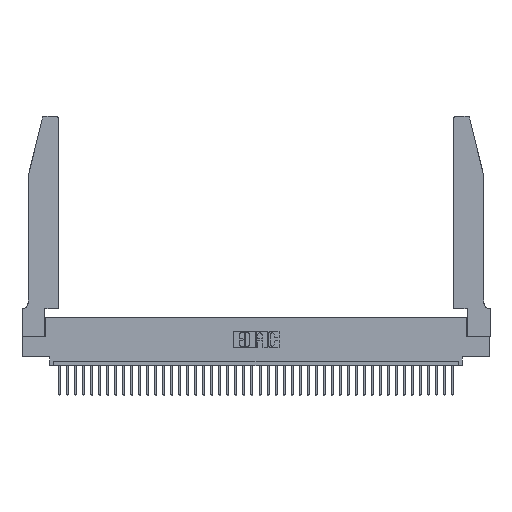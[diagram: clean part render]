
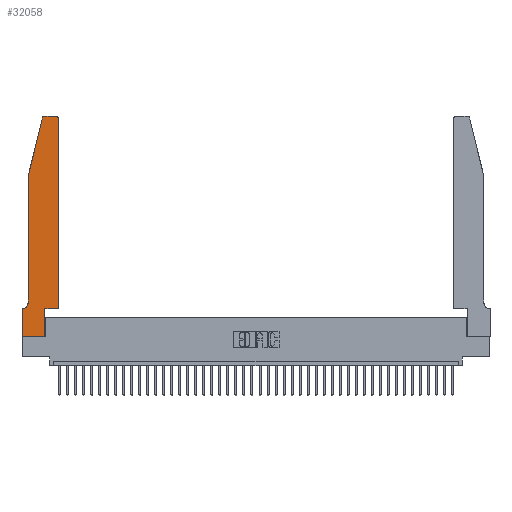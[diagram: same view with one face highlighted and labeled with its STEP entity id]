
A CAD part, top view. The second image highlights one B-rep face of the part: STEP entity #32058.
In plain terms, the highlighted planar face has unit normal (0, 0, 1).
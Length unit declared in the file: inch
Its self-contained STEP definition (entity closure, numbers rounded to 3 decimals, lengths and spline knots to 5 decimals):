
#206 = EDGE_CURVE ( 'NONE', #25502, #33551, #23242, .T. ) ;
#455 = VERTEX_POINT ( 'NONE', #18061 ) ;
#619 = VECTOR ( 'NONE', #20736, 39.37008 ) ;
#912 = EDGE_CURVE ( 'NONE', #34437, #13391, #27772, .T. ) ;
#1024 = ORIENTED_EDGE ( 'NONE', *, *, #29469, .T. ) ;
#1064 = VECTOR ( 'NONE', #20770, 39.37008 ) ;
#1552 = CARTESIAN_POINT ( 'NONE',  ( 0.2605, 2.75, 0.37 ) ) ;
#1917 = VECTOR ( 'NONE', #2538, 39.37008 ) ;
#2538 = DIRECTION ( 'NONE',  ( 0., -1., 0. ) ) ;
#2721 = VERTEX_POINT ( 'NONE', #35830 ) ;
#3305 = DIRECTION ( 'NONE',  ( 0., 0., 1. ) ) ;
#3306 = ORIENTED_EDGE ( 'NONE', *, *, #912, .T. ) ;
#3746 = CARTESIAN_POINT ( 'NONE',  ( 0., 0.35, 0.37 ) ) ;
#4103 = EDGE_CURVE ( 'NONE', #31707, #2721, #30834, .T. ) ;
#4588 = ORIENTED_EDGE ( 'NONE', *, *, #35322, .T. ) ;
#5431 = EDGE_CURVE ( 'NONE', #2721, #13974, #35699, .T. ) ;
#6191 = EDGE_CURVE ( 'NONE', #33551, #34437, #24695, .T. ) ;
#6424 = LINE ( 'NONE', #40690, #1917 ) ;
#6462 = CARTESIAN_POINT ( 'NONE',  ( 0.25487, 2.72718, 0.37 ) ) ;
#6508 = PLANE ( 'NONE',  #7336 ) ;
#7336 = AXIS2_PLACEMENT_3D ( 'NONE', #16289, #38538, #25572 ) ;
#8213 = CARTESIAN_POINT ( 'NONE',  ( 0.4205, 2.75, 0.37 ) ) ;
#9357 = LINE ( 'NONE', #32837, #37346 ) ;
#9524 = FACE_OUTER_BOUND ( 'NONE', #13750, .T. ) ;
#9936 = CARTESIAN_POINT ( 'NONE',  ( 0.0055, 0.35, 0.37 ) ) ;
#10356 = VERTEX_POINT ( 'NONE', #9936 ) ;
#10572 = DIRECTION ( 'NONE',  ( 1., 0., 0. ) ) ;
#10891 = DIRECTION ( 'NONE',  ( -1., 0., 0. ) ) ;
#11150 = CARTESIAN_POINT ( 'NONE',  ( 0.0755, 0.35, 0.37 ) ) ;
#11899 = VECTOR ( 'NONE', #15461, 39.37008 ) ;
#12122 = EDGE_CURVE ( 'NONE', #10356, #31707, #17173, .T. ) ;
#12181 = VECTOR ( 'NONE', #20592, 39.37008 ) ;
#12443 = AXIS2_PLACEMENT_3D ( 'NONE', #22425, #17047, #10572 ) ;
#13391 = VERTEX_POINT ( 'NONE', #6462 ) ;
#13750 = EDGE_LOOP ( 'NONE', ( #18812, #3306, #4588, #18172, #1024, #31462, #36913, #40579, #20035, #32049, #25837, #37815 ) ) ;
#13974 = VERTEX_POINT ( 'NONE', #38502 ) ;
#14275 = AXIS2_PLACEMENT_3D ( 'NONE', #18850, #3305, #25412 ) ;
#14450 = CARTESIAN_POINT ( 'NONE',  ( 0.0755, 2., 0.37 ) ) ;
#14494 = VECTOR ( 'NONE', #14606, 39.37008 ) ;
#14606 = DIRECTION ( 'NONE',  ( 0., 1., 0. ) ) ;
#15461 = DIRECTION ( 'NONE',  ( 1., 0., 0. ) ) ;
#16007 = VERTEX_POINT ( 'NONE', #33804 ) ;
#16289 = CARTESIAN_POINT ( 'NONE',  ( 0., 0.35, 0.37 ) ) ;
#16657 = LINE ( 'NONE', #14450, #12181 ) ;
#17047 = DIRECTION ( 'NONE',  ( 0., 0., 1. ) ) ;
#17173 = LINE ( 'NONE', #11150, #34203 ) ;
#17203 = DIRECTION ( 'NONE',  ( 0., 1., 0. ) ) ;
#18061 = CARTESIAN_POINT ( 'NONE',  ( 0.4505, 0.35, 0.37 ) ) ;
#18172 = ORIENTED_EDGE ( 'NONE', *, *, #33239, .T. ) ;
#18812 = ORIENTED_EDGE ( 'NONE', *, *, #6191, .T. ) ;
#18850 = CARTESIAN_POINT ( 'NONE',  ( 0.284, 2.72, 0.37 ) ) ;
#19788 = DIRECTION ( 'NONE',  ( -1., 0., 0. ) ) ;
#20035 = ORIENTED_EDGE ( 'NONE', *, *, #40458, .T. ) ;
#20268 = VECTOR ( 'NONE', #29416, 39.37008 ) ;
#20376 = AXIS2_PLACEMENT_3D ( 'NONE', #36208, #27139, #10891 ) ;
#20592 = DIRECTION ( 'NONE',  ( -0.239, -0.971, 0. ) ) ;
#20736 = DIRECTION ( 'NONE',  ( 1., 0., 0. ) ) ;
#20770 = DIRECTION ( 'NONE',  ( -1., 0., 0. ) ) ;
#21089 = VERTEX_POINT ( 'NONE', #29851 ) ;
#21393 = CARTESIAN_POINT ( 'NONE',  ( 0., 0., 0.37 ) ) ;
#22425 = CARTESIAN_POINT ( 'NONE',  ( 0.4205, 2.72, 0.37 ) ) ;
#22738 = CARTESIAN_POINT ( 'NONE',  ( 0., 0., 0.37 ) ) ;
#23242 = CIRCLE ( 'NONE', #12443, 0.03 ) ;
#24695 = LINE ( 'NONE', #1552, #1064 ) ;
#24753 = CARTESIAN_POINT ( 'NONE',  ( 0.284, 2.75, 0.37 ) ) ;
#25395 = CARTESIAN_POINT ( 'NONE',  ( 0.4505, 0.35, 0.37 ) ) ;
#25412 = DIRECTION ( 'NONE',  ( 1., 0., 0. ) ) ;
#25502 = VERTEX_POINT ( 'NONE', #31188 ) ;
#25572 = DIRECTION ( 'NONE',  ( 1., 0., 0. ) ) ;
#25837 = ORIENTED_EDGE ( 'NONE', *, *, #32381, .T. ) ;
#26734 = CARTESIAN_POINT ( 'NONE',  ( 0.0755, 2., 0.37 ) ) ;
#27139 = DIRECTION ( 'NONE',  ( 0., 0., -1. ) ) ;
#27772 = CIRCLE ( 'NONE', #14275, 0.03 ) ;
#28534 = VERTEX_POINT ( 'NONE', #26734 ) ;
#29416 = DIRECTION ( 'NONE',  ( 0., -1., 0. ) ) ;
#29469 = EDGE_CURVE ( 'NONE', #21089, #10356, #30207, .T. ) ;
#29851 = CARTESIAN_POINT ( 'NONE',  ( 0.0755, 0.42, 0.37 ) ) ;
#30207 = CIRCLE ( 'NONE', #20376, 0.07 ) ;
#30834 = LINE ( 'NONE', #22738, #20268 ) ;
#31188 = CARTESIAN_POINT ( 'NONE',  ( 0.4505, 2.72, 0.37 ) ) ;
#31462 = ORIENTED_EDGE ( 'NONE', *, *, #12122, .T. ) ;
#31707 = VERTEX_POINT ( 'NONE', #3746 ) ;
#32049 = ORIENTED_EDGE ( 'NONE', *, *, #40186, .T. ) ;
#32058 = ADVANCED_FACE ( 'NONE', ( #9524 ), #6508, .T. ) ;
#32381 = EDGE_CURVE ( 'NONE', #455, #25502, #32487, .T. ) ;
#32487 = LINE ( 'NONE', #33741, #14494 ) ;
#32837 = CARTESIAN_POINT ( 'NONE',  ( 0.2865, 0.35, 0.37 ) ) ;
#33239 = EDGE_CURVE ( 'NONE', #28534, #21089, #6424, .T. ) ;
#33551 = VERTEX_POINT ( 'NONE', #8213 ) ;
#33741 = CARTESIAN_POINT ( 'NONE',  ( 0.4505, 0.35, 0.37 ) ) ;
#33804 = CARTESIAN_POINT ( 'NONE',  ( 0.2865, 0.35, 0.37 ) ) ;
#34203 = VECTOR ( 'NONE', #19788, 39.37008 ) ;
#34437 = VERTEX_POINT ( 'NONE', #24753 ) ;
#35322 = EDGE_CURVE ( 'NONE', #13391, #28534, #16657, .T. ) ;
#35699 = LINE ( 'NONE', #21393, #619 ) ;
#35830 = CARTESIAN_POINT ( 'NONE',  ( 0., 0., 0.37 ) ) ;
#36208 = CARTESIAN_POINT ( 'NONE',  ( 0.0055, 0.42, 0.37 ) ) ;
#36913 = ORIENTED_EDGE ( 'NONE', *, *, #4103, .T. ) ;
#37346 = VECTOR ( 'NONE', #17203, 39.37008 ) ;
#37815 = ORIENTED_EDGE ( 'NONE', *, *, #206, .T. ) ;
#38416 = LINE ( 'NONE', #25395, #11899 ) ;
#38502 = CARTESIAN_POINT ( 'NONE',  ( 0.2865, 0., 0.37 ) ) ;
#38538 = DIRECTION ( 'NONE',  ( 0., 0., 1. ) ) ;
#40186 = EDGE_CURVE ( 'NONE', #16007, #455, #38416, .T. ) ;
#40458 = EDGE_CURVE ( 'NONE', #13974, #16007, #9357, .T. ) ;
#40579 = ORIENTED_EDGE ( 'NONE', *, *, #5431, .T. ) ;
#40690 = CARTESIAN_POINT ( 'NONE',  ( 0.0755, 2., 0.37 ) ) ;
